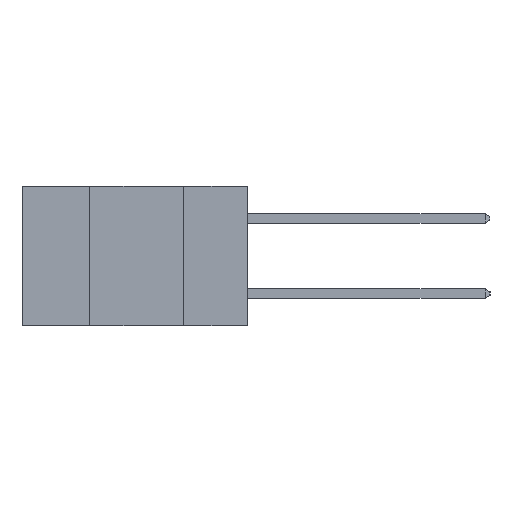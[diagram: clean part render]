
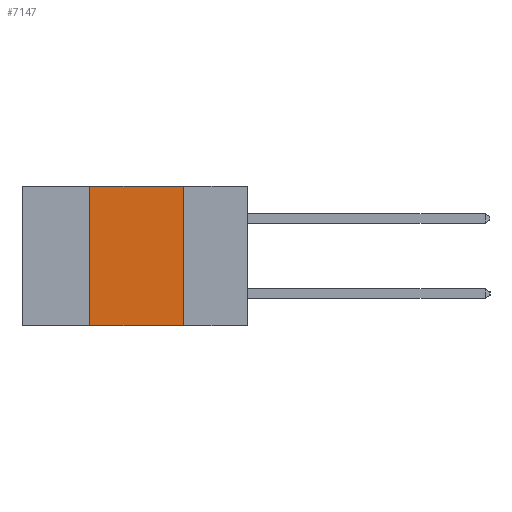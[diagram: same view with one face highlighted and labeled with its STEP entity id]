
A CAD part, left-side view. The second image highlights one B-rep face of the part: STEP entity #7147.
In plain terms, the highlighted planar face has unit normal (-1, 0, 0).
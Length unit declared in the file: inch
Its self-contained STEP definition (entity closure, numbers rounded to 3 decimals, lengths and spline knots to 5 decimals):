
#380 = LINE ( 'NONE', #15541, #1147 ) ;
#825 = ORIENTED_EDGE ( 'NONE', *, *, #8423, .T. ) ;
#907 = CARTESIAN_POINT ( 'NONE',  ( 0., 0.42, 0. ) ) ;
#1147 = VECTOR ( 'NONE', #15373, 39.37008 ) ;
#2972 = ORIENTED_EDGE ( 'NONE', *, *, #4220, .F. ) ;
#3345 = ORIENTED_EDGE ( 'NONE', *, *, #6697, .F. ) ;
#3366 = EDGE_CURVE ( 'NONE', #5698, #13697, #15367, .T. ) ;
#4220 = EDGE_CURVE ( 'NONE', #13965, #5698, #380, .T. ) ;
#5698 = VERTEX_POINT ( 'NONE', #7562 ) ;
#5983 = CARTESIAN_POINT ( 'NONE',  ( 0., 0.42, -0.37 ) ) ;
#6697 = EDGE_CURVE ( 'NONE', #9174, #13965, #7195, .T. ) ;
#7147 = ADVANCED_FACE ( 'NONE', ( #13829 ), #14480, .F. ) ;
#7195 = LINE ( 'NONE', #10959, #14226 ) ;
#7547 = VECTOR ( 'NONE', #9412, 39.37008 ) ;
#7562 = CARTESIAN_POINT ( 'NONE',  ( 0., 0.17, 0. ) ) ;
#7844 = CARTESIAN_POINT ( 'NONE',  ( 0., 0.17, -0.37 ) ) ;
#8423 = EDGE_CURVE ( 'NONE', #9174, #13697, #12819, .T. ) ;
#8645 = AXIS2_PLACEMENT_3D ( 'NONE', #14427, #15383, #15215 ) ;
#8654 = ORIENTED_EDGE ( 'NONE', *, *, #3366, .F. ) ;
#8819 = VECTOR ( 'NONE', #11357, 39.37008 ) ;
#9118 = CARTESIAN_POINT ( 'NONE',  ( 0., 0.6, -0.37 ) ) ;
#9174 = VERTEX_POINT ( 'NONE', #5983 ) ;
#9412 = DIRECTION ( 'NONE',  ( 0., -1., 0. ) ) ;
#10758 = DIRECTION ( 'NONE',  ( 0., 0., 1. ) ) ;
#10959 = CARTESIAN_POINT ( 'NONE',  ( 0., 0.42, -0.37 ) ) ;
#11357 = DIRECTION ( 'NONE',  ( 0., 0., -1. ) ) ;
#11394 = CARTESIAN_POINT ( 'NONE',  ( 0., 0.17, -0.37 ) ) ;
#11794 = EDGE_LOOP ( 'NONE', ( #8654, #2972, #3345, #825 ) ) ;
#12819 = LINE ( 'NONE', #9118, #7547 ) ;
#13697 = VERTEX_POINT ( 'NONE', #7844 ) ;
#13829 = FACE_OUTER_BOUND ( 'NONE', #11794, .T. ) ;
#13965 = VERTEX_POINT ( 'NONE', #907 ) ;
#14226 = VECTOR ( 'NONE', #10758, 39.37008 ) ;
#14427 = CARTESIAN_POINT ( 'NONE',  ( 0., 0.6, 0. ) ) ;
#14480 = PLANE ( 'NONE',  #8645 ) ;
#15215 = DIRECTION ( 'NONE',  ( 0., 0., -1. ) ) ;
#15367 = LINE ( 'NONE', #11394, #8819 ) ;
#15373 = DIRECTION ( 'NONE',  ( 0., -1., 0. ) ) ;
#15383 = DIRECTION ( 'NONE',  ( 1., 0., 0. ) ) ;
#15541 = CARTESIAN_POINT ( 'NONE',  ( 0., 0.6, 0. ) ) ;
